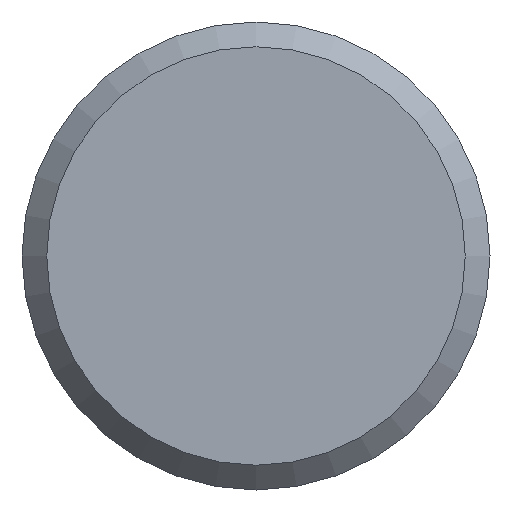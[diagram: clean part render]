
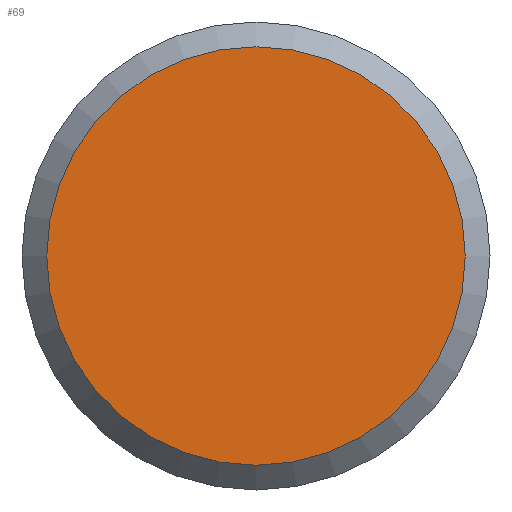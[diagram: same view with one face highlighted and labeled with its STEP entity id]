
A CAD part, left-side view. The second image highlights one B-rep face of the part: STEP entity #69.
In plain terms, the highlighted planar face has unit normal (-1, 0, 0).
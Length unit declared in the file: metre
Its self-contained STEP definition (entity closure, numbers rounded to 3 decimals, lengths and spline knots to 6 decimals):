
#69 = ADVANCED_FACE( '', ( #149 ), #150, .T. );
#149 = FACE_OUTER_BOUND( '', #230, .T. );
#150 = PLANE( '', #231 );
#230 = EDGE_LOOP( '', ( #331 ) );
#231 = AXIS2_PLACEMENT_3D( '', #332, #333, #334 );
#331 = ORIENTED_EDGE( '', *, *, #391, .F. );
#332 = CARTESIAN_POINT( '', ( 0., 0., 0. ) );
#333 = DIRECTION( '', ( -1., 0., 0. ) );
#334 = DIRECTION( '', ( 0., -1., 0. ) );
#391 = EDGE_CURVE( '', #443, #443, #444, .T. );
#443 = VERTEX_POINT( '', #498 );
#444 = CIRCLE( '', #499, 0.004293 );
#498 = CARTESIAN_POINT( '', ( 0., 0.004293, 0. ) );
#499 = AXIS2_PLACEMENT_3D( '', #557, #558, #559 );
#557 = CARTESIAN_POINT( '', ( 0., 0., 0. ) );
#558 = DIRECTION( '', ( 1., 0., 0. ) );
#559 = DIRECTION( '', ( 0., 1., 0. ) );
